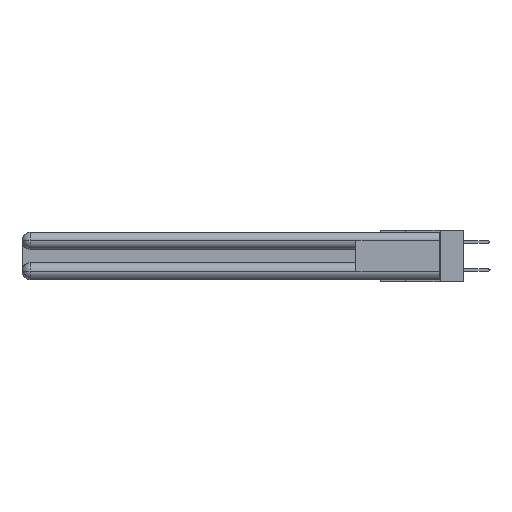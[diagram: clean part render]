
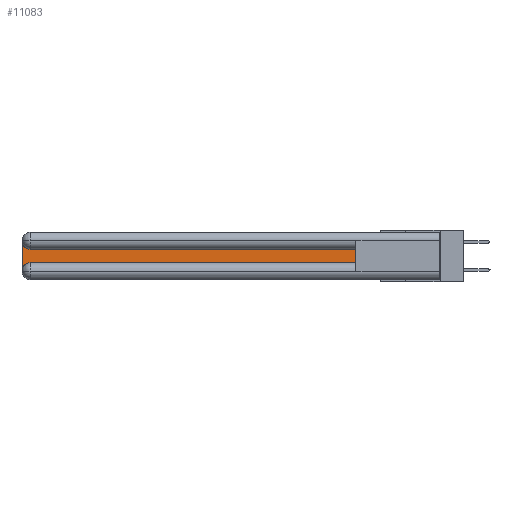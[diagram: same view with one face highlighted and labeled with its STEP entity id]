
A CAD part, left-side view. The second image highlights one B-rep face of the part: STEP entity #11083.
In plain terms, the highlighted planar face has unit normal (-1, 0, 0).
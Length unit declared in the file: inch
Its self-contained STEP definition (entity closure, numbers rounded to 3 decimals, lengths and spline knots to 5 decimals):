
#304 = CARTESIAN_POINT ( 'NONE',  ( 0.075, 3., -0.0625 ) ) ;
#1858 = CARTESIAN_POINT ( 'NONE',  ( 0.075, 0.6, -0.1225 ) ) ;
#2442 = EDGE_LOOP ( 'NONE', ( #9493, #3787, #11613, #24256, #8289, #26637 ) ) ;
#2640 = CARTESIAN_POINT ( 'NONE',  ( 0.075, 2.94, -0.1225 ) ) ;
#3497 = FACE_OUTER_BOUND ( 'NONE', #2442, .T. ) ;
#3498 = AXIS2_PLACEMENT_3D ( 'NONE', #27126, #19464, #5118 ) ;
#3670 = CIRCLE ( 'NONE', #15791, 0.06 ) ;
#3749 = DIRECTION ( 'NONE',  ( 0., -1., 0. ) ) ;
#3787 = ORIENTED_EDGE ( 'NONE', *, *, #12393, .T. ) ;
#3931 = CARTESIAN_POINT ( 'NONE',  ( 0.075, 0.6, -0.2175 ) ) ;
#3958 = CARTESIAN_POINT ( 'NONE',  ( 0.075, 0.6, -0.2175 ) ) ;
#4910 = AXIS2_PLACEMENT_3D ( 'NONE', #12254, #24434, #17312 ) ;
#5118 = DIRECTION ( 'NONE',  ( 0., 0., -1. ) ) ;
#5549 = DIRECTION ( 'NONE',  ( 1., 0., 0. ) ) ;
#6725 = CIRCLE ( 'NONE', #4910, 0.06 ) ;
#7096 = EDGE_CURVE ( 'NONE', #31204, #20134, #12536, .T. ) ;
#7675 = DIRECTION ( 'NONE',  ( 0., 0., -1. ) ) ;
#8289 = ORIENTED_EDGE ( 'NONE', *, *, #27033, .T. ) ;
#9493 = ORIENTED_EDGE ( 'NONE', *, *, #7096, .T. ) ;
#10928 = VERTEX_POINT ( 'NONE', #304 ) ;
#11083 = ADVANCED_FACE ( 'NONE', ( #3497 ), #26803, .F. ) ;
#11613 = ORIENTED_EDGE ( 'NONE', *, *, #11658, .T. ) ;
#11658 = EDGE_CURVE ( 'NONE', #10928, #23756, #18194, .T. ) ;
#12254 = CARTESIAN_POINT ( 'NONE',  ( 0.075, 2.94, -0.2775 ) ) ;
#12393 = EDGE_CURVE ( 'NONE', #20134, #10928, #3670, .T. ) ;
#12536 = LINE ( 'NONE', #14770, #22881 ) ;
#12608 = CARTESIAN_POINT ( 'NONE',  ( 0.075, 3., -0.2775 ) ) ;
#12694 = EDGE_CURVE ( 'NONE', #16943, #31204, #17015, .T. ) ;
#12752 = VECTOR ( 'NONE', #3749, 39.37008 ) ;
#12768 = VECTOR ( 'NONE', #25815, 39.37008 ) ;
#13278 = CARTESIAN_POINT ( 'NONE',  ( 0.075, 2.94, -0.2175 ) ) ;
#14770 = CARTESIAN_POINT ( 'NONE',  ( 0.075, 0.6, -0.1225 ) ) ;
#14816 = VERTEX_POINT ( 'NONE', #13278 ) ;
#14878 = DIRECTION ( 'NONE',  ( 0., 1., 0. ) ) ;
#15120 = CARTESIAN_POINT ( 'NONE',  ( 0.075, 0.6, -0.2175 ) ) ;
#15791 = AXIS2_PLACEMENT_3D ( 'NONE', #27239, #5549, #7675 ) ;
#16679 = CARTESIAN_POINT ( 'NONE',  ( 0.075, 3., -0.2175 ) ) ;
#16943 = VERTEX_POINT ( 'NONE', #15120 ) ;
#17015 = LINE ( 'NONE', #3931, #12768 ) ;
#17312 = DIRECTION ( 'NONE',  ( 0., 0., -1. ) ) ;
#18194 = LINE ( 'NONE', #16679, #18956 ) ;
#18903 = LINE ( 'NONE', #3958, #12752 ) ;
#18956 = VECTOR ( 'NONE', #19138, 39.37008 ) ;
#19138 = DIRECTION ( 'NONE',  ( 0., 0., -1. ) ) ;
#19464 = DIRECTION ( 'NONE',  ( 1., 0., 0. ) ) ;
#20134 = VERTEX_POINT ( 'NONE', #2640 ) ;
#21260 = EDGE_CURVE ( 'NONE', #23756, #14816, #6725, .T. ) ;
#22881 = VECTOR ( 'NONE', #14878, 39.37008 ) ;
#23756 = VERTEX_POINT ( 'NONE', #12608 ) ;
#24256 = ORIENTED_EDGE ( 'NONE', *, *, #21260, .T. ) ;
#24434 = DIRECTION ( 'NONE',  ( 1., 0., 0. ) ) ;
#25815 = DIRECTION ( 'NONE',  ( 0., 0., 1. ) ) ;
#26637 = ORIENTED_EDGE ( 'NONE', *, *, #12694, .T. ) ;
#26803 = PLANE ( 'NONE',  #3498 ) ;
#27033 = EDGE_CURVE ( 'NONE', #14816, #16943, #18903, .T. ) ;
#27126 = CARTESIAN_POINT ( 'NONE',  ( 0.075, 3., -0.1225 ) ) ;
#27239 = CARTESIAN_POINT ( 'NONE',  ( 0.075, 2.94, -0.0625 ) ) ;
#31204 = VERTEX_POINT ( 'NONE', #1858 ) ;
